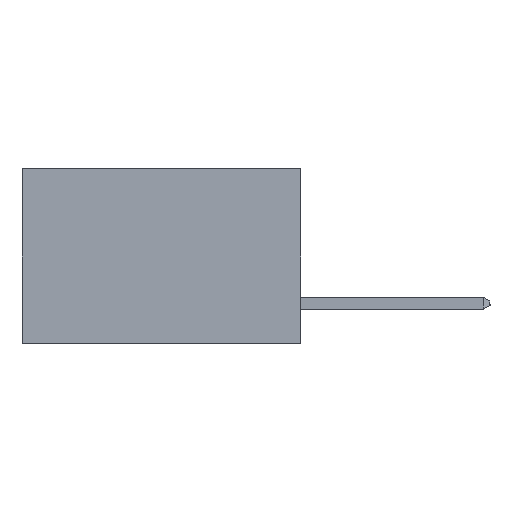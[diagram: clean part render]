
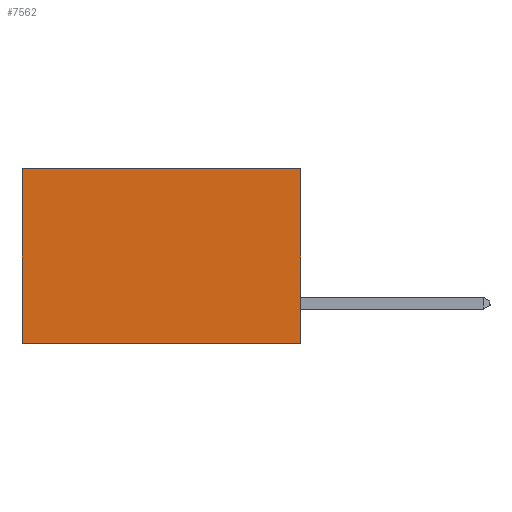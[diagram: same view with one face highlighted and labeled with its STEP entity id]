
A CAD part, left-side view. The second image highlights one B-rep face of the part: STEP entity #7562.
In plain terms, the highlighted planar face has unit normal (-1, 0, 0).
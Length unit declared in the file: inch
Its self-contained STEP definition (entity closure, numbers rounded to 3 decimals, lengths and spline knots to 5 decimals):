
#206 = VECTOR ( 'NONE', #995, 39.37008 ) ;
#505 = CARTESIAN_POINT ( 'NONE',  ( 0.277, 0.59, -0.37 ) ) ;
#763 = DIRECTION ( 'NONE',  ( 0., 0., -1. ) ) ;
#812 = VERTEX_POINT ( 'NONE', #4213 ) ;
#950 = CARTESIAN_POINT ( 'NONE',  ( 0.277, 0.59, 0. ) ) ;
#995 = DIRECTION ( 'NONE',  ( 0., 0., -1. ) ) ;
#1540 = EDGE_CURVE ( 'NONE', #812, #7533, #9974, .T. ) ;
#1615 = ORIENTED_EDGE ( 'NONE', *, *, #1540, .F. ) ;
#2051 = DIRECTION ( 'NONE',  ( 0., 1., 0. ) ) ;
#2662 = LINE ( 'NONE', #505, #2940 ) ;
#2711 = CARTESIAN_POINT ( 'NONE',  ( 0.277, 0., -0.37 ) ) ;
#2940 = VECTOR ( 'NONE', #11254, 39.37008 ) ;
#3035 = CARTESIAN_POINT ( 'NONE',  ( 0.277, 0., 0. ) ) ;
#3451 = FACE_OUTER_BOUND ( 'NONE', #4311, .T. ) ;
#3534 = PLANE ( 'NONE',  #8930 ) ;
#3659 = VERTEX_POINT ( 'NONE', #950 ) ;
#3785 = LINE ( 'NONE', #3035, #7853 ) ;
#4213 = CARTESIAN_POINT ( 'NONE',  ( 0.277, 0., -0.37 ) ) ;
#4311 = EDGE_LOOP ( 'NONE', ( #10444, #1615, #11078, #7041 ) ) ;
#4726 = VERTEX_POINT ( 'NONE', #5714 ) ;
#4975 = EDGE_CURVE ( 'NONE', #4726, #812, #7411, .T. ) ;
#5514 = EDGE_CURVE ( 'NONE', #4726, #3659, #3785, .T. ) ;
#5554 = EDGE_CURVE ( 'NONE', #3659, #7533, #2662, .T. ) ;
#5714 = CARTESIAN_POINT ( 'NONE',  ( 0.277, 0., 0. ) ) ;
#6230 = DIRECTION ( 'NONE',  ( 1., 0., 0. ) ) ;
#6398 = CARTESIAN_POINT ( 'NONE',  ( 0.277, 0., -0.37 ) ) ;
#7041 = ORIENTED_EDGE ( 'NONE', *, *, #5514, .T. ) ;
#7411 = LINE ( 'NONE', #2711, #206 ) ;
#7533 = VERTEX_POINT ( 'NONE', #8674 ) ;
#7562 = ADVANCED_FACE ( 'NONE', ( #3451 ), #3534, .F. ) ;
#7739 = VECTOR ( 'NONE', #9680, 39.37008 ) ;
#7853 = VECTOR ( 'NONE', #2051, 39.37008 ) ;
#8674 = CARTESIAN_POINT ( 'NONE',  ( 0.277, 0.59, -0.37 ) ) ;
#8930 = AXIS2_PLACEMENT_3D ( 'NONE', #11194, #6230, #763 ) ;
#9680 = DIRECTION ( 'NONE',  ( 0., 1., 0. ) ) ;
#9974 = LINE ( 'NONE', #6398, #7739 ) ;
#10444 = ORIENTED_EDGE ( 'NONE', *, *, #5554, .T. ) ;
#11078 = ORIENTED_EDGE ( 'NONE', *, *, #4975, .F. ) ;
#11194 = CARTESIAN_POINT ( 'NONE',  ( 0.277, 0., -0.37 ) ) ;
#11254 = DIRECTION ( 'NONE',  ( 0., 0., -1. ) ) ;
